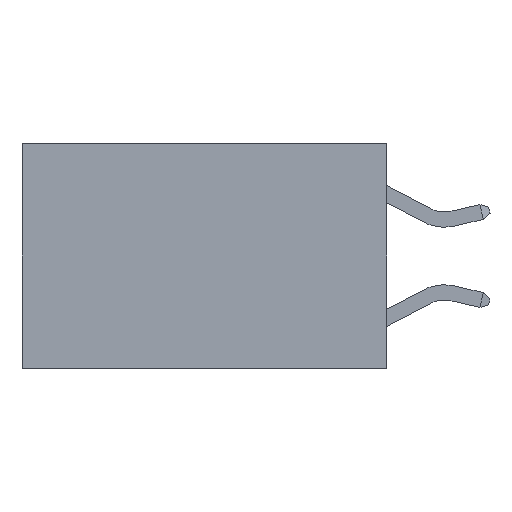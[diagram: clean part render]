
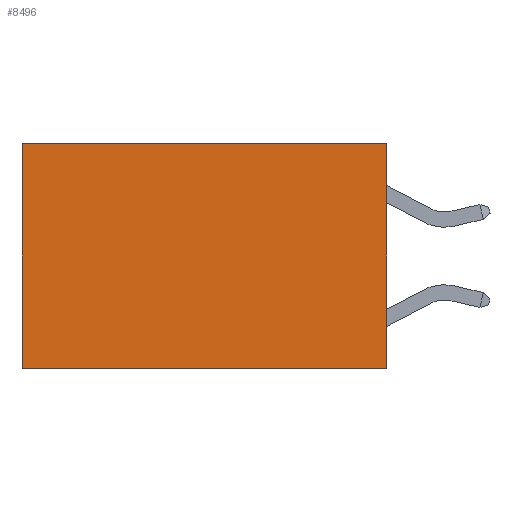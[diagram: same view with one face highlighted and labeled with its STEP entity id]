
A CAD part, left-side view. The second image highlights one B-rep face of the part: STEP entity #8496.
In plain terms, the highlighted planar face has unit normal (-1, 0, 0).
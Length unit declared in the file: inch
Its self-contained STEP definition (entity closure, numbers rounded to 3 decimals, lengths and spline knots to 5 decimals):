
#189 = ORIENTED_EDGE ( 'NONE', *, *, #7383, .T. ) ;
#1090 = FACE_OUTER_BOUND ( 'NONE', #3255, .T. ) ;
#1192 = EDGE_CURVE ( 'NONE', #1750, #2682, #9139, .T. ) ;
#1750 = VERTEX_POINT ( 'NONE', #3004 ) ;
#2183 = VERTEX_POINT ( 'NONE', #9685 ) ;
#2268 = ORIENTED_EDGE ( 'NONE', *, *, #7304, .F. ) ;
#2451 = DIRECTION ( 'NONE',  ( 0., 1., 0. ) ) ;
#2682 = VERTEX_POINT ( 'NONE', #6185 ) ;
#3004 = CARTESIAN_POINT ( 'NONE',  ( 0.2625, 0., -0.37 ) ) ;
#3128 = AXIS2_PLACEMENT_3D ( 'NONE', #10143, #9412, #7844 ) ;
#3228 = LINE ( 'NONE', #7556, #5996 ) ;
#3255 = EDGE_LOOP ( 'NONE', ( #189, #10948, #2268, #4335 ) ) ;
#3908 = VECTOR ( 'NONE', #4032, 39.37008 ) ;
#4032 = DIRECTION ( 'NONE',  ( 0., 0., -1. ) ) ;
#4335 = ORIENTED_EDGE ( 'NONE', *, *, #6471, .T. ) ;
#4680 = VECTOR ( 'NONE', #9683, 39.37008 ) ;
#4950 = LINE ( 'NONE', #8904, #4680 ) ;
#5010 = DIRECTION ( 'NONE',  ( 0., 1., 0. ) ) ;
#5041 = VECTOR ( 'NONE', #5010, 39.37008 ) ;
#5682 = CARTESIAN_POINT ( 'NONE',  ( 0.2625, 0.6, 0. ) ) ;
#5996 = VECTOR ( 'NONE', #2451, 39.37008 ) ;
#6109 = CARTESIAN_POINT ( 'NONE',  ( 0.2625, 0., -0.37 ) ) ;
#6121 = LINE ( 'NONE', #5682, #3908 ) ;
#6171 = PLANE ( 'NONE',  #3128 ) ;
#6185 = CARTESIAN_POINT ( 'NONE',  ( 0.2625, 0.6, -0.37 ) ) ;
#6471 = EDGE_CURVE ( 'NONE', #2183, #6497, #3228, .T. ) ;
#6497 = VERTEX_POINT ( 'NONE', #8379 ) ;
#7304 = EDGE_CURVE ( 'NONE', #2183, #1750, #4950, .T. ) ;
#7383 = EDGE_CURVE ( 'NONE', #6497, #2682, #6121, .T. ) ;
#7556 = CARTESIAN_POINT ( 'NONE',  ( 0.2625, 0., 0. ) ) ;
#7844 = DIRECTION ( 'NONE',  ( 0., 0., -1. ) ) ;
#8379 = CARTESIAN_POINT ( 'NONE',  ( 0.2625, 0.6, 0. ) ) ;
#8496 = ADVANCED_FACE ( 'NONE', ( #1090 ), #6171, .F. ) ;
#8904 = CARTESIAN_POINT ( 'NONE',  ( 0.2625, 0., 0. ) ) ;
#9139 = LINE ( 'NONE', #6109, #5041 ) ;
#9412 = DIRECTION ( 'NONE',  ( 1., 0., 0. ) ) ;
#9683 = DIRECTION ( 'NONE',  ( 0., 0., -1. ) ) ;
#9685 = CARTESIAN_POINT ( 'NONE',  ( 0.2625, 0., 0. ) ) ;
#10143 = CARTESIAN_POINT ( 'NONE',  ( 0.2625, 0., 0. ) ) ;
#10948 = ORIENTED_EDGE ( 'NONE', *, *, #1192, .F. ) ;
